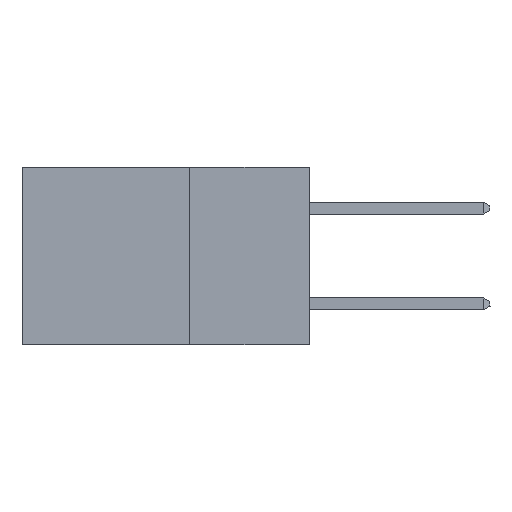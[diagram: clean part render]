
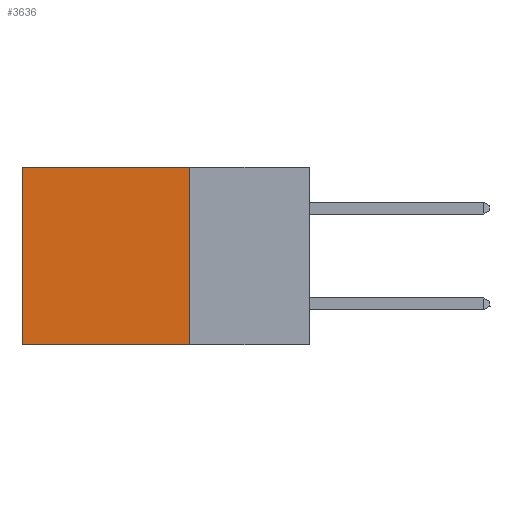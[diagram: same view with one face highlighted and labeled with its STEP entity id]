
A CAD part, left-side view. The second image highlights one B-rep face of the part: STEP entity #3636.
In plain terms, the highlighted planar face has unit normal (-1, 0, 0).
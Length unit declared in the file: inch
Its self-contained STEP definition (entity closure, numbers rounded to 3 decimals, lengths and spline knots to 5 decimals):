
#6 = CARTESIAN_POINT ( 'NONE',  ( 0.2875, 0.6, 0. ) ) ;
#1201 = DIRECTION ( 'NONE',  ( 1., 0., 0. ) ) ;
#1514 = VECTOR ( 'NONE', #31107, 39.37008 ) ;
#2594 = CARTESIAN_POINT ( 'NONE',  ( 0.2875, 0.25, 0. ) ) ;
#2851 = VERTEX_POINT ( 'NONE', #18561 ) ;
#2881 = CARTESIAN_POINT ( 'NONE',  ( 0.2875, 0.25, 0. ) ) ;
#3636 = ADVANCED_FACE ( 'NONE', ( #17699 ), #30197, .F. ) ;
#3826 = EDGE_CURVE ( 'NONE', #5742, #9434, #19432, .T. ) ;
#5742 = VERTEX_POINT ( 'NONE', #6 ) ;
#6333 = ORIENTED_EDGE ( 'NONE', *, *, #3826, .T. ) ;
#6873 = LINE ( 'NONE', #31426, #32093 ) ;
#7128 = ORIENTED_EDGE ( 'NONE', *, *, #21416, .F. ) ;
#7697 = CARTESIAN_POINT ( 'NONE',  ( 0.2875, 0.25, 0. ) ) ;
#9434 = VERTEX_POINT ( 'NONE', #19649 ) ;
#10627 = ORIENTED_EDGE ( 'NONE', *, *, #23019, .T. ) ;
#14153 = ORIENTED_EDGE ( 'NONE', *, *, #17953, .F. ) ;
#14359 = DIRECTION ( 'NONE',  ( 0., 1., 0. ) ) ;
#17155 = DIRECTION ( 'NONE',  ( 0., 0., -1. ) ) ;
#17699 = FACE_OUTER_BOUND ( 'NONE', #31408, .T. ) ;
#17803 = LINE ( 'NONE', #7697, #22607 ) ;
#17953 = EDGE_CURVE ( 'NONE', #2851, #21490, #17803, .T. ) ;
#18561 = CARTESIAN_POINT ( 'NONE',  ( 0.2875, 0.25, 0. ) ) ;
#19166 = VECTOR ( 'NONE', #27158, 39.37008 ) ;
#19432 = LINE ( 'NONE', #26538, #1514 ) ;
#19649 = CARTESIAN_POINT ( 'NONE',  ( 0.2875, 0.6, -0.37 ) ) ;
#19692 = AXIS2_PLACEMENT_3D ( 'NONE', #2881, #1201, #19999 ) ;
#19999 = DIRECTION ( 'NONE',  ( 0., 0., -1. ) ) ;
#21416 = EDGE_CURVE ( 'NONE', #21490, #9434, #6873, .T. ) ;
#21490 = VERTEX_POINT ( 'NONE', #31199 ) ;
#22607 = VECTOR ( 'NONE', #17155, 39.37008 ) ;
#23019 = EDGE_CURVE ( 'NONE', #2851, #5742, #29766, .T. ) ;
#26538 = CARTESIAN_POINT ( 'NONE',  ( 0.2875, 0.6, 0. ) ) ;
#27158 = DIRECTION ( 'NONE',  ( 0., 1., 0. ) ) ;
#29766 = LINE ( 'NONE', #2594, #19166 ) ;
#30197 = PLANE ( 'NONE',  #19692 ) ;
#31107 = DIRECTION ( 'NONE',  ( 0., 0., -1. ) ) ;
#31199 = CARTESIAN_POINT ( 'NONE',  ( 0.2875, 0.25, -0.37 ) ) ;
#31408 = EDGE_LOOP ( 'NONE', ( #6333, #7128, #14153, #10627 ) ) ;
#31426 = CARTESIAN_POINT ( 'NONE',  ( 0.2875, 0.25, -0.37 ) ) ;
#32093 = VECTOR ( 'NONE', #14359, 39.37008 ) ;
